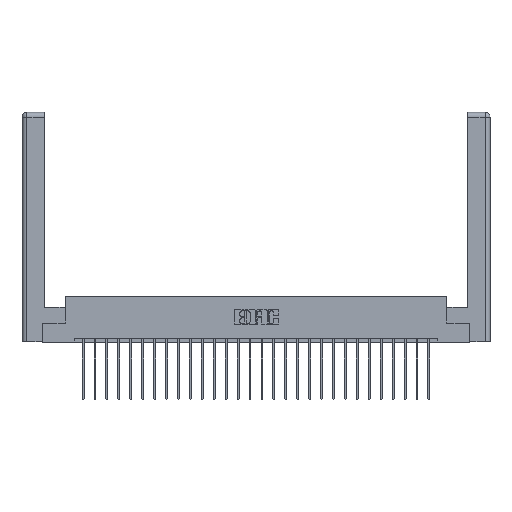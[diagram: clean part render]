
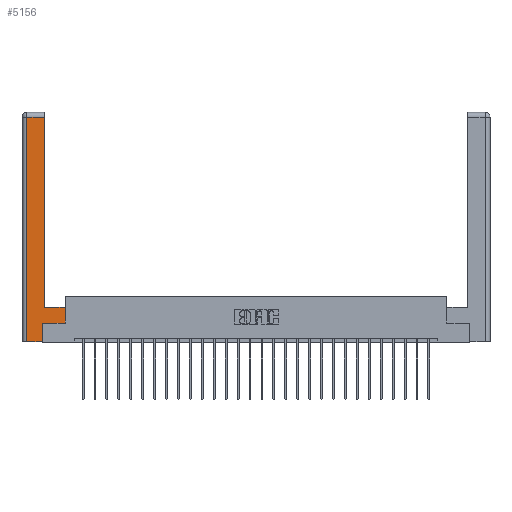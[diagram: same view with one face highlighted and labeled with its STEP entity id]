
A CAD part, top view. The second image highlights one B-rep face of the part: STEP entity #5156.
In plain terms, the highlighted planar face has unit normal (0, 0, 1).
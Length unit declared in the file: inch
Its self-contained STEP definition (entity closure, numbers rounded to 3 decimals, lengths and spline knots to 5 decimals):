
#93 = DIRECTION ( 'NONE',  ( -1., 0., 0. ) ) ;
#96 = CARTESIAN_POINT ( 'NONE',  ( 0.295, 3., 0. ) ) ;
#238 = VECTOR ( 'NONE', #7813, 39.37008 ) ;
#609 = AXIS2_PLACEMENT_3D ( 'NONE', #4664, #13238, #19539 ) ;
#997 = CARTESIAN_POINT ( 'NONE',  ( 0.0615, 2.94, 0. ) ) ;
#1112 = VERTEX_POINT ( 'NONE', #14672 ) ;
#1353 = CARTESIAN_POINT ( 'NONE',  ( 0.0615, 2.94, 0. ) ) ;
#1680 = LINE ( 'NONE', #4050, #17948 ) ;
#1915 = VECTOR ( 'NONE', #9446, 39.37008 ) ;
#2026 = VECTOR ( 'NONE', #21411, 39.37008 ) ;
#4050 = CARTESIAN_POINT ( 'NONE',  ( 0.0615, 0., 0. ) ) ;
#4664 = CARTESIAN_POINT ( 'NONE',  ( 0., 0., 0. ) ) ;
#5156 = ADVANCED_FACE ( 'NONE', ( #26970 ), #17393, .F. ) ;
#5739 = ORIENTED_EDGE ( 'NONE', *, *, #5891, .T. ) ;
#5891 = EDGE_CURVE ( 'NONE', #17112, #21699, #1680, .T. ) ;
#5927 = LINE ( 'NONE', #997, #1915 ) ;
#6121 = VERTEX_POINT ( 'NONE', #7051 ) ;
#6290 = DIRECTION ( 'NONE',  ( 0., 1., 0. ) ) ;
#6401 = ORIENTED_EDGE ( 'NONE', *, *, #8839, .T. ) ;
#6491 = DIRECTION ( 'NONE',  ( 0., 1., 0. ) ) ;
#6742 = CARTESIAN_POINT ( 'NONE',  ( 0.0615, 0., 0. ) ) ;
#6753 = CARTESIAN_POINT ( 'NONE',  ( 0.295, 0.45, 0. ) ) ;
#7051 = CARTESIAN_POINT ( 'NONE',  ( 0.295, 2.94, 0. ) ) ;
#7369 = ORIENTED_EDGE ( 'NONE', *, *, #24510, .T. ) ;
#7813 = DIRECTION ( 'NONE',  ( 1., 0., 0. ) ) ;
#8594 = ORIENTED_EDGE ( 'NONE', *, *, #20394, .T. ) ;
#8839 = EDGE_CURVE ( 'NONE', #21699, #14863, #20628, .T. ) ;
#9345 = CARTESIAN_POINT ( 'NONE',  ( 0.265, 0., 0. ) ) ;
#9446 = DIRECTION ( 'NONE',  ( -1., 0., 0. ) ) ;
#9757 = CARTESIAN_POINT ( 'NONE',  ( 0.565, 0.245, 0. ) ) ;
#10033 = ORIENTED_EDGE ( 'NONE', *, *, #23742, .T. ) ;
#11112 = ORIENTED_EDGE ( 'NONE', *, *, #26874, .T. ) ;
#11575 = VECTOR ( 'NONE', #6491, 39.37008 ) ;
#11768 = ORIENTED_EDGE ( 'NONE', *, *, #20574, .T. ) ;
#12470 = CARTESIAN_POINT ( 'NONE',  ( 0.565, 0.45, 0. ) ) ;
#13052 = VECTOR ( 'NONE', #93, 39.37008 ) ;
#13073 = LINE ( 'NONE', #12470, #18715 ) ;
#13238 = DIRECTION ( 'NONE',  ( 0., 0., -1. ) ) ;
#14443 = ORIENTED_EDGE ( 'NONE', *, *, #21527, .T. ) ;
#14672 = CARTESIAN_POINT ( 'NONE',  ( 0.565, 0.45, 0. ) ) ;
#14863 = VERTEX_POINT ( 'NONE', #9345 ) ;
#14944 = CARTESIAN_POINT ( 'NONE',  ( 0.265, 0., 0. ) ) ;
#15612 = CARTESIAN_POINT ( 'NONE',  ( 0.265, 0.245, 0. ) ) ;
#16238 = LINE ( 'NONE', #9757, #238 ) ;
#16916 = CARTESIAN_POINT ( 'NONE',  ( 0.565, 0.245, 0. ) ) ;
#17112 = VERTEX_POINT ( 'NONE', #1353 ) ;
#17393 = PLANE ( 'NONE',  #609 ) ;
#17745 = CARTESIAN_POINT ( 'NONE',  ( 0.265, 0.245, 0. ) ) ;
#17906 = DIRECTION ( 'NONE',  ( 0., 1., 0. ) ) ;
#17948 = VECTOR ( 'NONE', #21114, 39.37008 ) ;
#18715 = VECTOR ( 'NONE', #6290, 39.37008 ) ;
#19539 = DIRECTION ( 'NONE',  ( -1., 0., 0. ) ) ;
#20394 = EDGE_CURVE ( 'NONE', #14863, #22098, #22653, .T. ) ;
#20574 = EDGE_CURVE ( 'NONE', #1112, #22891, #27335, .T. ) ;
#20628 = LINE ( 'NONE', #14944, #2026 ) ;
#21114 = DIRECTION ( 'NONE',  ( 0., -1., 0. ) ) ;
#21411 = DIRECTION ( 'NONE',  ( 1., 0., 0. ) ) ;
#21527 = EDGE_CURVE ( 'NONE', #26355, #1112, #13073, .T. ) ;
#21699 = VERTEX_POINT ( 'NONE', #6742 ) ;
#22098 = VERTEX_POINT ( 'NONE', #15612 ) ;
#22653 = LINE ( 'NONE', #17745, #26654 ) ;
#22891 = VERTEX_POINT ( 'NONE', #26195 ) ;
#23742 = EDGE_CURVE ( 'NONE', #22891, #6121, #24514, .T. ) ;
#24510 = EDGE_CURVE ( 'NONE', #22098, #26355, #16238, .T. ) ;
#24514 = LINE ( 'NONE', #96, #11575 ) ;
#26195 = CARTESIAN_POINT ( 'NONE',  ( 0.295, 0.45, 0. ) ) ;
#26355 = VERTEX_POINT ( 'NONE', #16916 ) ;
#26654 = VECTOR ( 'NONE', #17906, 39.37008 ) ;
#26874 = EDGE_CURVE ( 'NONE', #6121, #17112, #5927, .T. ) ;
#26970 = FACE_OUTER_BOUND ( 'NONE', #27284, .T. ) ;
#27284 = EDGE_LOOP ( 'NONE', ( #10033, #11112, #5739, #6401, #8594, #7369, #14443, #11768 ) ) ;
#27335 = LINE ( 'NONE', #6753, #13052 ) ;
